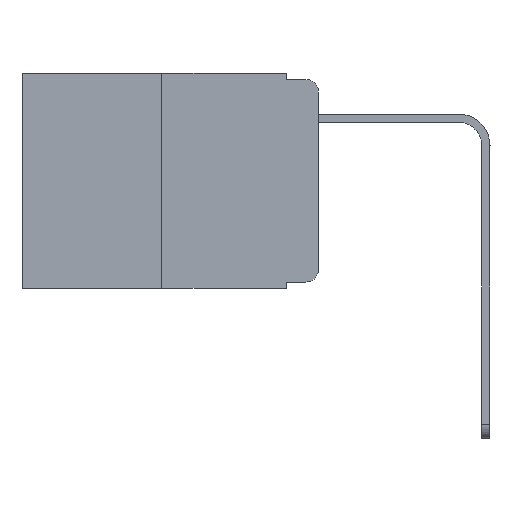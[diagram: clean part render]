
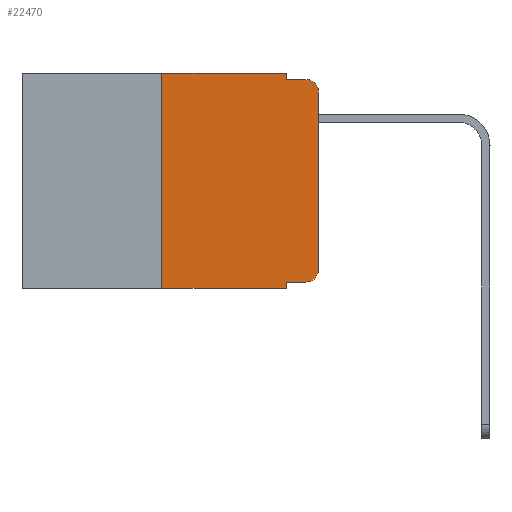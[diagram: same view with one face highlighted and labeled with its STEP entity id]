
A CAD part, left-side view. The second image highlights one B-rep face of the part: STEP entity #22470.
In plain terms, the highlighted planar face has unit normal (-1, 0, 0).
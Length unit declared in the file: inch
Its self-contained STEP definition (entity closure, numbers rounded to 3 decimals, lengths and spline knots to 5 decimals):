
#184 = EDGE_CURVE ( 'NONE', #20060, #3990, #10355, .T. ) ;
#477 = DIRECTION ( 'NONE',  ( 0., 0., -1. ) ) ;
#734 = EDGE_CURVE ( 'NONE', #2419, #3990, #18329, .T. ) ;
#964 = CARTESIAN_POINT ( 'NONE',  ( 0., 0.051, -0.01 ) ) ;
#977 = CARTESIAN_POINT ( 'NONE',  ( 0., 0.02, -0.313 ) ) ;
#1655 = VERTEX_POINT ( 'NONE', #11281 ) ;
#1840 = CARTESIAN_POINT ( 'NONE',  ( 0., 0.02, -0.03 ) ) ;
#2156 = VECTOR ( 'NONE', #14443, 39.37008 ) ;
#2267 = EDGE_CURVE ( 'NONE', #12386, #14365, #10264, .T. ) ;
#2419 = VERTEX_POINT ( 'NONE', #964 ) ;
#2508 = VECTOR ( 'NONE', #22228, 39.37008 ) ;
#2604 = CARTESIAN_POINT ( 'NONE',  ( 0., 0.25, 0. ) ) ;
#2840 = DIRECTION ( 'NONE',  ( 0., 0., 1. ) ) ;
#3243 = DIRECTION ( 'NONE',  ( -1., 0., 0. ) ) ;
#3351 = LINE ( 'NONE', #19709, #19106 ) ;
#3456 = VECTOR ( 'NONE', #13308, 39.37008 ) ;
#3478 = FACE_OUTER_BOUND ( 'NONE', #13054, .T. ) ;
#3990 = VERTEX_POINT ( 'NONE', #5837 ) ;
#4046 = CARTESIAN_POINT ( 'NONE',  ( 0., 0.473, 0. ) ) ;
#4815 = VECTOR ( 'NONE', #12979, 39.37008 ) ;
#5659 = EDGE_CURVE ( 'NONE', #10412, #14365, #15473, .T. ) ;
#5837 = CARTESIAN_POINT ( 'NONE',  ( 0., 0.02, -0.01 ) ) ;
#6394 = LINE ( 'NONE', #12481, #9972 ) ;
#6581 = CARTESIAN_POINT ( 'NONE',  ( 0., 0.051, 0. ) ) ;
#6778 = VERTEX_POINT ( 'NONE', #6581 ) ;
#7539 = EDGE_CURVE ( 'NONE', #1655, #20060, #17602, .T. ) ;
#7668 = CIRCLE ( 'NONE', #18180, 0.02 ) ;
#8162 = AXIS2_PLACEMENT_3D ( 'NONE', #1840, #14239, #10470 ) ;
#8465 = ORIENTED_EDGE ( 'NONE', *, *, #19030, .F. ) ;
#8550 = CARTESIAN_POINT ( 'NONE',  ( 0., 0.473, -0.343 ) ) ;
#9972 = VECTOR ( 'NONE', #10694, 39.37008 ) ;
#10031 = ORIENTED_EDGE ( 'NONE', *, *, #2267, .T. ) ;
#10264 = LINE ( 'NONE', #8550, #12750 ) ;
#10355 = CIRCLE ( 'NONE', #8162, 0.02 ) ;
#10412 = VERTEX_POINT ( 'NONE', #20679 ) ;
#10470 = DIRECTION ( 'NONE',  ( 0., 0., -1. ) ) ;
#10694 = DIRECTION ( 'NONE',  ( 0., -1., 0. ) ) ;
#11086 = VERTEX_POINT ( 'NONE', #13714 ) ;
#11118 = PLANE ( 'NONE',  #13611 ) ;
#11177 = ORIENTED_EDGE ( 'NONE', *, *, #5659, .F. ) ;
#11281 = CARTESIAN_POINT ( 'NONE',  ( 0., 0., -0.313 ) ) ;
#12386 = VERTEX_POINT ( 'NONE', #17623 ) ;
#12481 = CARTESIAN_POINT ( 'NONE',  ( 0., 0.051, -0.333 ) ) ;
#12685 = CARTESIAN_POINT ( 'NONE',  ( 0., 0., 0. ) ) ;
#12738 = CARTESIAN_POINT ( 'NONE',  ( 0., 0., -0.03 ) ) ;
#12750 = VECTOR ( 'NONE', #20948, 39.37008 ) ;
#12979 = DIRECTION ( 'NONE',  ( 0., -1., 0. ) ) ;
#13054 = EDGE_LOOP ( 'NONE', ( #17176, #20322, #14423, #18297, #13384, #8465, #10031, #11177, #13314, #22031 ) ) ;
#13308 = DIRECTION ( 'NONE',  ( 0., -1., 0. ) ) ;
#13314 = ORIENTED_EDGE ( 'NONE', *, *, #18885, .T. ) ;
#13384 = ORIENTED_EDGE ( 'NONE', *, *, #13419, .F. ) ;
#13419 = EDGE_CURVE ( 'NONE', #11086, #6778, #14182, .T. ) ;
#13426 = CARTESIAN_POINT ( 'NONE',  ( 0., 0.02, -0.333 ) ) ;
#13611 = AXIS2_PLACEMENT_3D ( 'NONE', #4046, #19957, #477 ) ;
#13714 = CARTESIAN_POINT ( 'NONE',  ( 0., 0.25, 0. ) ) ;
#14182 = LINE ( 'NONE', #16792, #3456 ) ;
#14239 = DIRECTION ( 'NONE',  ( -1., 0., 0. ) ) ;
#14365 = VERTEX_POINT ( 'NONE', #17615 ) ;
#14423 = ORIENTED_EDGE ( 'NONE', *, *, #734, .F. ) ;
#14443 = DIRECTION ( 'NONE',  ( 0., 0., 1. ) ) ;
#15227 = VECTOR ( 'NONE', #2840, 39.37008 ) ;
#15232 = CARTESIAN_POINT ( 'NONE',  ( 0., 0.051, 0. ) ) ;
#15473 = LINE ( 'NONE', #15232, #2508 ) ;
#16192 = EDGE_CURVE ( 'NONE', #6778, #2419, #3351, .T. ) ;
#16426 = DIRECTION ( 'NONE',  ( 0., 0., -1. ) ) ;
#16476 = CARTESIAN_POINT ( 'NONE',  ( 0., 0.051, -0.01 ) ) ;
#16792 = CARTESIAN_POINT ( 'NONE',  ( 0., 0.473, 0. ) ) ;
#17176 = ORIENTED_EDGE ( 'NONE', *, *, #7539, .T. ) ;
#17602 = LINE ( 'NONE', #12685, #2156 ) ;
#17615 = CARTESIAN_POINT ( 'NONE',  ( 0., 0.051, -0.343 ) ) ;
#17623 = CARTESIAN_POINT ( 'NONE',  ( 0., 0.25, -0.343 ) ) ;
#18180 = AXIS2_PLACEMENT_3D ( 'NONE', #977, #3243, #20798 ) ;
#18297 = ORIENTED_EDGE ( 'NONE', *, *, #16192, .F. ) ;
#18329 = LINE ( 'NONE', #16476, #4815 ) ;
#18885 = EDGE_CURVE ( 'NONE', #10412, #20250, #6394, .T. ) ;
#19030 = EDGE_CURVE ( 'NONE', #12386, #11086, #21635, .T. ) ;
#19106 = VECTOR ( 'NONE', #16426, 39.37008 ) ;
#19709 = CARTESIAN_POINT ( 'NONE',  ( 0., 0.051, 0. ) ) ;
#19957 = DIRECTION ( 'NONE',  ( 1., 0., 0. ) ) ;
#20060 = VERTEX_POINT ( 'NONE', #12738 ) ;
#20250 = VERTEX_POINT ( 'NONE', #13426 ) ;
#20322 = ORIENTED_EDGE ( 'NONE', *, *, #184, .T. ) ;
#20679 = CARTESIAN_POINT ( 'NONE',  ( 0., 0.051, -0.333 ) ) ;
#20753 = EDGE_CURVE ( 'NONE', #20250, #1655, #7668, .T. ) ;
#20798 = DIRECTION ( 'NONE',  ( 0., 0., -1. ) ) ;
#20948 = DIRECTION ( 'NONE',  ( 0., -1., 0. ) ) ;
#21635 = LINE ( 'NONE', #2604, #15227 ) ;
#22031 = ORIENTED_EDGE ( 'NONE', *, *, #20753, .T. ) ;
#22228 = DIRECTION ( 'NONE',  ( 0., 0., -1. ) ) ;
#22470 = ADVANCED_FACE ( 'NONE', ( #3478 ), #11118, .F. ) ;
